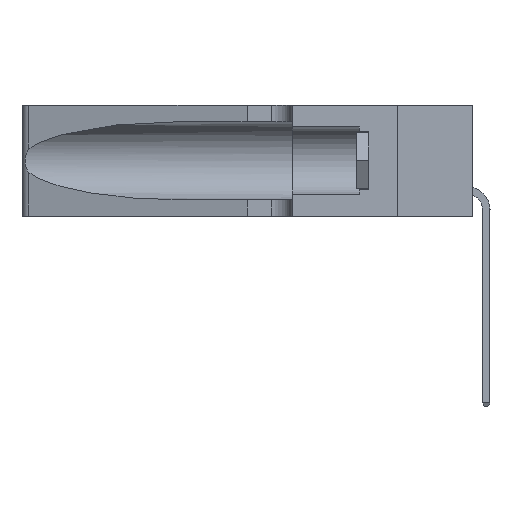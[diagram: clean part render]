
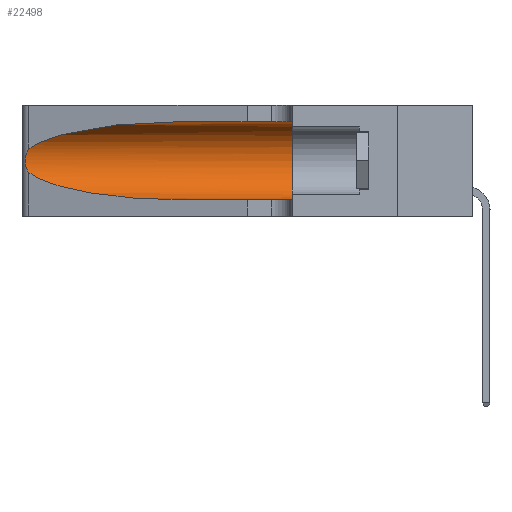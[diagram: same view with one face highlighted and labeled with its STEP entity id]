
A CAD part, left-side view. The second image highlights one B-rep face of the part: STEP entity #22498.
In plain terms, the highlighted cylindrical face has radius 3.308 mm (diameter 6.617 mm), a partial arc.
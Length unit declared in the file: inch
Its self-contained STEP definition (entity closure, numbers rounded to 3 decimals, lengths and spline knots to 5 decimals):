
#705 = EDGE_CURVE ( 'NONE', #17378, #23686, #47758, .T. ) ;
#1178 = CARTESIAN_POINT ( 'NONE',  ( 0.25555, 1.22994, 0.2215 ) ) ;
#1838 = CARTESIAN_POINT ( 'NONE',  ( 0.26075, 1.23896, 0.19203 ) ) ;
#1974 = CARTESIAN_POINT ( 'NONE',  ( 0.25555, 1.22993, 0.14849 ) ) ;
#2322 = AXIS2_PLACEMENT_3D ( 'NONE', #5855, #31857, #46092 ) ;
#3816 = VERTEX_POINT ( 'NONE', #16540 ) ;
#4261 = EDGE_CURVE ( 'NONE', #46496, #3816, #29672, .T. ) ;
#4637 = LINE ( 'NONE', #34202, #13442 ) ;
#5388 = CARTESIAN_POINT ( 'NONE',  ( 0.25487, 1.22718, 0.22369 ) ) ;
#5562 = CARTESIAN_POINT ( 'NONE',  ( 0.26017, 1.23833, 0.17102 ) ) ;
#5855 = CARTESIAN_POINT ( 'NONE',  ( 0.1305, 0.35, 0.185 ) ) ;
#6119 = LINE ( 'NONE', #25826, #17105 ) ;
#7298 = ORIENTED_EDGE ( 'NONE', *, *, #8083, .F. ) ;
#7836 = DIRECTION ( 'NONE',  ( 0., -1., 0. ) ) ;
#8083 = EDGE_CURVE ( 'NONE', #35460, #29681, #28699, .T. ) ;
#8631 = CARTESIAN_POINT ( 'NONE',  ( 0.25854, 1.2359, 0.20912 ) ) ;
#8780 = B_SPLINE_CURVE_WITH_KNOTS ( 'NONE', 3,
 ( #5388, #1178, #12881, #27209, #8631, #34612, #1838, #27878, #5562, #12399, #19894, #23654, #1974, #42489 ),
 .UNSPECIFIED., .F., .F.,
 ( 4, 2, 2, 2, 2, 2, 4 ),
 ( 0., 0.00027, 0.00053, 0.00107, 0.0016, 0.00187, 0.00214 ),
 .UNSPECIFIED. ) ;
#10880 = CARTESIAN_POINT ( 'NONE',  ( 0.2373, 1.15595, 0.28018 ) ) ;
#11502 = CARTESIAN_POINT ( 'NONE',  ( 0.1305, 0.35, 0.31525 ) ) ;
#11711 = ORIENTED_EDGE ( 'NONE', *, *, #4261, .T. ) ;
#12399 = CARTESIAN_POINT ( 'NONE',  ( 0.25856, 1.23593, 0.16098 ) ) ;
#12493 = ORIENTED_EDGE ( 'NONE', *, *, #25877, .T. ) ;
#12881 = CARTESIAN_POINT ( 'NONE',  ( 0.25639, 1.23184, 0.21858 ) ) ;
#13442 = VECTOR ( 'NONE', #22750, 39.37008 ) ;
#14180 = CARTESIAN_POINT ( 'NONE',  ( 0.25487, 1.22718, 0.22369 ) ) ;
#14404 = DIRECTION ( 'NONE',  ( 0., -1., 0. ) ) ;
#15781 = CARTESIAN_POINT ( 'NONE',  ( 0.25487, 1.22718, 0.14631 ) ) ;
#16540 = CARTESIAN_POINT ( 'NONE',  ( 0.25487, 1.22718, 0.22369 ) ) ;
#17105 = VECTOR ( 'NONE', #14404, 39.37008 ) ;
#17378 = VERTEX_POINT ( 'NONE', #43260 ) ;
#19894 = CARTESIAN_POINT ( 'NONE',  ( 0.25789, 1.23486, 0.15765 ) ) ;
#21331 = CARTESIAN_POINT ( 'NONE',  ( 0.1305, 0.72297, 0.05475 ) ) ;
#21380 = CYLINDRICAL_SURFACE ( 'NONE', #35648, 0.13025 ) ;
#21920 = FACE_OUTER_BOUND ( 'NONE', #46750, .T. ) ;
#22166 = CARTESIAN_POINT ( 'NONE',  ( 0.18966, 0.96281, 0.31525 ) ) ;
#22498 = ADVANCED_FACE ( 'NONE', ( #21920 ), #21380, .F. ) ;
#22750 = DIRECTION ( 'NONE',  ( 0., -1., 0. ) ) ;
#23654 = CARTESIAN_POINT ( 'NONE',  ( 0.25639, 1.23186, 0.15144 ) ) ;
#23686 = VERTEX_POINT ( 'NONE', #21331 ) ;
#25826 = CARTESIAN_POINT ( 'NONE',  ( 0.1305, 1.61858, 0.31525 ) ) ;
#25877 = EDGE_CURVE ( 'NONE', #3816, #17378, #8780, .T. ) ;
#26725 = CARTESIAN_POINT ( 'NONE',  ( 0.2373, 1.15595, 0.08982 ) ) ;
#27064 = CARTESIAN_POINT ( 'NONE',  ( 0.18966, 0.96281, 0.05475 ) ) ;
#27209 = CARTESIAN_POINT ( 'NONE',  ( 0.25787, 1.23484, 0.2124 ) ) ;
#27878 = CARTESIAN_POINT ( 'NONE',  ( 0.26075, 1.23896, 0.178 ) ) ;
#28699 = CIRCLE ( 'NONE', #2322, 0.13025 ) ;
#29672 =( BOUNDED_CURVE ( )  B_SPLINE_CURVE ( 3, ( #47879, #22166, #10880, #14180 ),
 .UNSPECIFIED., .F., .F. ) 
 B_SPLINE_CURVE_WITH_KNOTS ( ( 4, 4 ),
 ( 1.5708, 2.84003 ),
 .UNSPECIFIED. ) 
 CURVE ( )  GEOMETRIC_REPRESENTATION_ITEM ( )  RATIONAL_B_SPLINE_CURVE ( ( 1., 0.87, 0.87, 1. ) ) 
 REPRESENTATION_ITEM ( '' )  );
#29681 = VERTEX_POINT ( 'NONE', #47430 ) ;
#30257 = ORIENTED_EDGE ( 'NONE', *, *, #36565, .T. ) ;
#31027 = CARTESIAN_POINT ( 'NONE',  ( 0.1305, 0.72297, 0.31525 ) ) ;
#31857 = DIRECTION ( 'NONE',  ( 0., 1., 0. ) ) ;
#33984 = DIRECTION ( 'NONE',  ( 0., 0., -1. ) ) ;
#34202 = CARTESIAN_POINT ( 'NONE',  ( 0.1305, 1.61858, 0.05475 ) ) ;
#34612 = CARTESIAN_POINT ( 'NONE',  ( 0.26018, 1.23835, 0.19895 ) ) ;
#35460 = VERTEX_POINT ( 'NONE', #11502 ) ;
#35648 = AXIS2_PLACEMENT_3D ( 'NONE', #40649, #7836, #33984 ) ;
#35849 = ORIENTED_EDGE ( 'NONE', *, *, #42244, .F. ) ;
#36565 = EDGE_CURVE ( 'NONE', #23686, #29681, #4637, .T. ) ;
#37871 = CARTESIAN_POINT ( 'NONE',  ( 0.1305, 0.72297, 0.05475 ) ) ;
#40649 = CARTESIAN_POINT ( 'NONE',  ( 0.1305, 1.61858, 0.185 ) ) ;
#42244 = EDGE_CURVE ( 'NONE', #46496, #35460, #6119, .T. ) ;
#42489 = CARTESIAN_POINT ( 'NONE',  ( 0.25487, 1.22718, 0.14631 ) ) ;
#43260 = CARTESIAN_POINT ( 'NONE',  ( 0.25487, 1.22718, 0.14631 ) ) ;
#45566 = ORIENTED_EDGE ( 'NONE', *, *, #705, .T. ) ;
#46092 = DIRECTION ( 'NONE',  ( 0., 0., 1. ) ) ;
#46496 = VERTEX_POINT ( 'NONE', #31027 ) ;
#46750 = EDGE_LOOP ( 'NONE', ( #11711, #12493, #45566, #30257, #7298, #35849 ) ) ;
#47430 = CARTESIAN_POINT ( 'NONE',  ( 0.1305, 0.35, 0.05475 ) ) ;
#47758 =( BOUNDED_CURVE ( )  B_SPLINE_CURVE ( 3, ( #15781, #26725, #27064, #37871 ),
 .UNSPECIFIED., .F., .T. ) 
 B_SPLINE_CURVE_WITH_KNOTS ( ( 4, 4 ),
 ( 3.44316, 4.71239 ),
 .UNSPECIFIED. ) 
 CURVE ( )  GEOMETRIC_REPRESENTATION_ITEM ( )  RATIONAL_B_SPLINE_CURVE ( ( 1., 0.87, 0.87, 1. ) ) 
 REPRESENTATION_ITEM ( '' )  );
#47879 = CARTESIAN_POINT ( 'NONE',  ( 0.1305, 0.72297, 0.31525 ) ) ;
